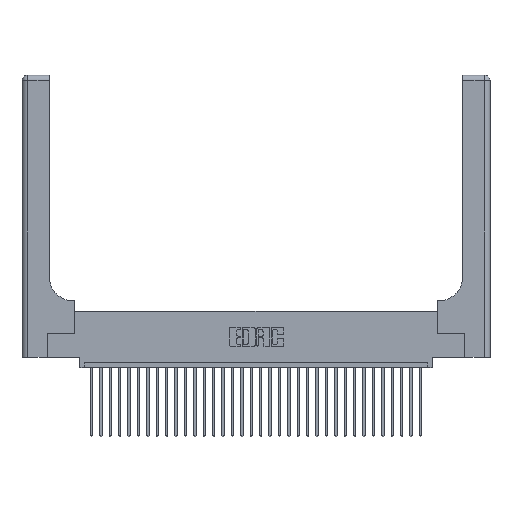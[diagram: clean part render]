
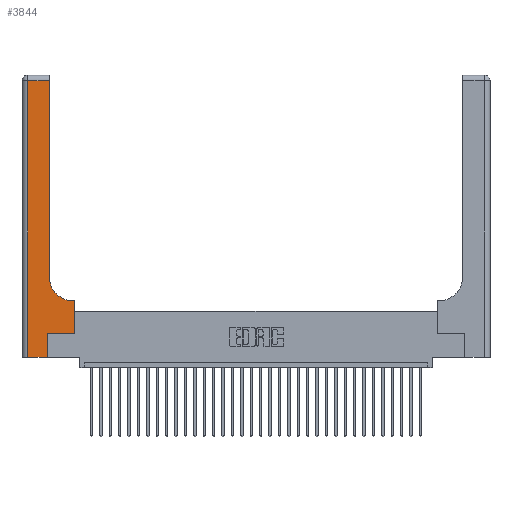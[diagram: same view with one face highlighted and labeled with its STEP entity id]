
A CAD part, top view. The second image highlights one B-rep face of the part: STEP entity #3844.
In plain terms, the highlighted planar face has unit normal (0, 0, 1).
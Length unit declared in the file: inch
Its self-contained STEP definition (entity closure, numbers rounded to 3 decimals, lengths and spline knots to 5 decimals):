
#704 = VECTOR ( 'NONE', #16662, 39.37008 ) ;
#897 = AXIS2_PLACEMENT_3D ( 'NONE', #26441, #26204, #11201 ) ;
#1490 = LINE ( 'NONE', #9799, #20677 ) ;
#1675 = VERTEX_POINT ( 'NONE', #6707 ) ;
#2067 = CARTESIAN_POINT ( 'NONE',  ( 0.2915, 2.94, 0.37 ) ) ;
#2515 = VECTOR ( 'NONE', #23458, 39.37008 ) ;
#3120 = LINE ( 'NONE', #5780, #20316 ) ;
#3318 = DIRECTION ( 'NONE',  ( 0., 1., 0. ) ) ;
#3470 = CARTESIAN_POINT ( 'NONE',  ( 0.269, 0.25, 0.37 ) ) ;
#3650 = CARTESIAN_POINT ( 'NONE',  ( 0., 2.94, 0.37 ) ) ;
#3844 = ADVANCED_FACE ( 'NONE', ( #6632 ), #21146, .F. ) ;
#3901 = VECTOR ( 'NONE', #17908, 39.37008 ) ;
#4746 = VECTOR ( 'NONE', #17620, 39.37008 ) ;
#5431 = CARTESIAN_POINT ( 'NONE',  ( 0., 0., 0.37 ) ) ;
#5474 = AXIS2_PLACEMENT_3D ( 'NONE', #14299, #24244, #16639 ) ;
#5780 = CARTESIAN_POINT ( 'NONE',  ( 0.269, 0., 0.37 ) ) ;
#6484 = CARTESIAN_POINT ( 'NONE',  ( 0.5585, 0.25, 0.37 ) ) ;
#6632 = FACE_OUTER_BOUND ( 'NONE', #7984, .T. ) ;
#6707 = CARTESIAN_POINT ( 'NONE',  ( 0.269, 0., 0.37 ) ) ;
#7984 = EDGE_LOOP ( 'NONE', ( #20498, #23073, #32623, #27991, #16172, #19291, #10728, #8588, #26054 ) ) ;
#8310 = LINE ( 'NONE', #3650, #704 ) ;
#8388 = CARTESIAN_POINT ( 'NONE',  ( 0.2915, 0.85, 0.37 ) ) ;
#8588 = ORIENTED_EDGE ( 'NONE', *, *, #22584, .T. ) ;
#9144 = EDGE_CURVE ( 'NONE', #26068, #16676, #30174, .T. ) ;
#9161 = DIRECTION ( 'NONE',  ( 1., 0., 0. ) ) ;
#9409 = EDGE_CURVE ( 'NONE', #15713, #19760, #13309, .T. ) ;
#9799 = CARTESIAN_POINT ( 'NONE',  ( 0.5585, 0.25, 0.37 ) ) ;
#9877 = CARTESIAN_POINT ( 'NONE',  ( 0.5585, 0.6, 0.37 ) ) ;
#10478 = LINE ( 'NONE', #3470, #12971 ) ;
#10728 = ORIENTED_EDGE ( 'NONE', *, *, #32003, .T. ) ;
#11201 = DIRECTION ( 'NONE',  ( -1., 0., 0. ) ) ;
#12771 = VERTEX_POINT ( 'NONE', #9877 ) ;
#12971 = VECTOR ( 'NONE', #9161, 39.37008 ) ;
#13309 = CIRCLE ( 'NONE', #5474, 0.25 ) ;
#13381 = EDGE_CURVE ( 'NONE', #16676, #1675, #29826, .T. ) ;
#14064 = EDGE_CURVE ( 'NONE', #19909, #19308, #10478, .T. ) ;
#14299 = CARTESIAN_POINT ( 'NONE',  ( 0.5415, 0.85, 0.37 ) ) ;
#15713 = VERTEX_POINT ( 'NONE', #17489 ) ;
#15927 = LINE ( 'NONE', #26061, #3901 ) ;
#16172 = ORIENTED_EDGE ( 'NONE', *, *, #25406, .T. ) ;
#16498 = VECTOR ( 'NONE', #22233, 39.37008 ) ;
#16639 = DIRECTION ( 'NONE',  ( 1., 0., 0. ) ) ;
#16662 = DIRECTION ( 'NONE',  ( -1., 0., 0. ) ) ;
#16667 = CARTESIAN_POINT ( 'NONE',  ( 0.06, 3., 0.37 ) ) ;
#16676 = VERTEX_POINT ( 'NONE', #24144 ) ;
#16863 = EDGE_CURVE ( 'NONE', #19760, #29030, #15927, .T. ) ;
#17241 = EDGE_CURVE ( 'NONE', #29030, #26068, #8310, .T. ) ;
#17489 = CARTESIAN_POINT ( 'NONE',  ( 0.5415, 0.6, 0.37 ) ) ;
#17620 = DIRECTION ( 'NONE',  ( -1., 0., 0. ) ) ;
#17908 = DIRECTION ( 'NONE',  ( 0., 1., 0. ) ) ;
#19163 = LINE ( 'NONE', #28014, #4746 ) ;
#19291 = ORIENTED_EDGE ( 'NONE', *, *, #14064, .T. ) ;
#19308 = VERTEX_POINT ( 'NONE', #6484 ) ;
#19760 = VERTEX_POINT ( 'NONE', #8388 ) ;
#19909 = VERTEX_POINT ( 'NONE', #22089 ) ;
#20316 = VECTOR ( 'NONE', #3318, 39.37008 ) ;
#20498 = ORIENTED_EDGE ( 'NONE', *, *, #16863, .T. ) ;
#20677 = VECTOR ( 'NONE', #32826, 39.37008 ) ;
#21146 = PLANE ( 'NONE',  #897 ) ;
#22089 = CARTESIAN_POINT ( 'NONE',  ( 0.269, 0.25, 0.37 ) ) ;
#22233 = DIRECTION ( 'NONE',  ( 0., -1., 0. ) ) ;
#22584 = EDGE_CURVE ( 'NONE', #12771, #15713, #19163, .T. ) ;
#23073 = ORIENTED_EDGE ( 'NONE', *, *, #17241, .T. ) ;
#23458 = DIRECTION ( 'NONE',  ( 1., 0., 0. ) ) ;
#24144 = CARTESIAN_POINT ( 'NONE',  ( 0.06, 0., 0.37 ) ) ;
#24244 = DIRECTION ( 'NONE',  ( 0., 0., -1. ) ) ;
#25406 = EDGE_CURVE ( 'NONE', #1675, #19909, #3120, .T. ) ;
#26054 = ORIENTED_EDGE ( 'NONE', *, *, #9409, .T. ) ;
#26061 = CARTESIAN_POINT ( 'NONE',  ( 0.2915, 3., 0.37 ) ) ;
#26068 = VERTEX_POINT ( 'NONE', #28729 ) ;
#26204 = DIRECTION ( 'NONE',  ( 0., 0., -1. ) ) ;
#26441 = CARTESIAN_POINT ( 'NONE',  ( 0., 3., 0.37 ) ) ;
#27991 = ORIENTED_EDGE ( 'NONE', *, *, #13381, .T. ) ;
#28014 = CARTESIAN_POINT ( 'NONE',  ( 0.2915, 0.6, 0.37 ) ) ;
#28729 = CARTESIAN_POINT ( 'NONE',  ( 0.06, 2.94, 0.37 ) ) ;
#29030 = VERTEX_POINT ( 'NONE', #2067 ) ;
#29826 = LINE ( 'NONE', #5431, #2515 ) ;
#30174 = LINE ( 'NONE', #16667, #16498 ) ;
#32003 = EDGE_CURVE ( 'NONE', #19308, #12771, #1490, .T. ) ;
#32623 = ORIENTED_EDGE ( 'NONE', *, *, #9144, .T. ) ;
#32826 = DIRECTION ( 'NONE',  ( 0., 1., 0. ) ) ;
